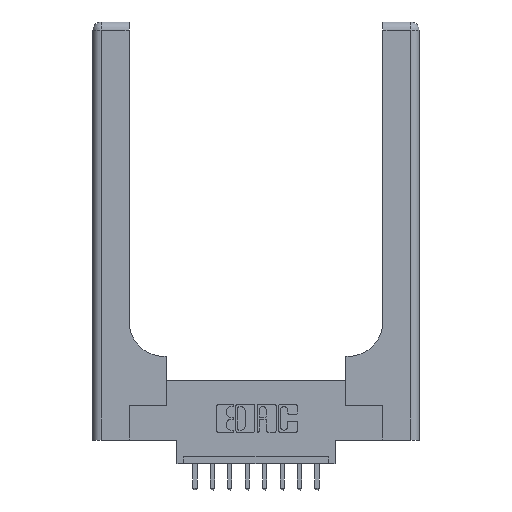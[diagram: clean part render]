
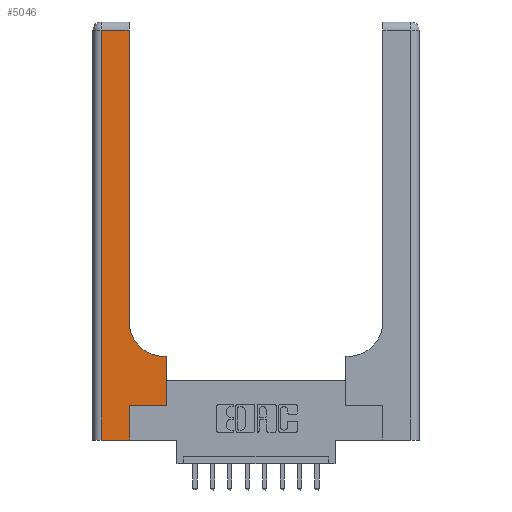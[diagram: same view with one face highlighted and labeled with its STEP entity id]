
A CAD part, top view. The second image highlights one B-rep face of the part: STEP entity #5046.
In plain terms, the highlighted planar face has unit normal (0, 0, 1).
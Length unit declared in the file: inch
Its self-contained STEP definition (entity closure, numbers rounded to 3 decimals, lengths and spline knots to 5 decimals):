
#338 = DIRECTION ( 'NONE',  ( 0., 0., -1. ) ) ;
#442 = ORIENTED_EDGE ( 'NONE', *, *, #2772, .T. ) ;
#544 = ORIENTED_EDGE ( 'NONE', *, *, #5323, .T. ) ;
#589 = VERTEX_POINT ( 'NONE', #1016 ) ;
#874 = VECTOR ( 'NONE', #15366, 39.37008 ) ;
#1016 = CARTESIAN_POINT ( 'NONE',  ( 0.51, 0.6, 0.37 ) ) ;
#1327 = DIRECTION ( 'NONE',  ( 1., 0., 0. ) ) ;
#1485 = VERTEX_POINT ( 'NONE', #12090 ) ;
#1653 = LINE ( 'NONE', #7400, #7604 ) ;
#1821 = VERTEX_POINT ( 'NONE', #3574 ) ;
#2405 = CARTESIAN_POINT ( 'NONE',  ( 0.265, 0.25, 0.37 ) ) ;
#2482 = LINE ( 'NONE', #2405, #5642 ) ;
#2516 = DIRECTION ( 'NONE',  ( 1., 0., 0. ) ) ;
#2554 = CARTESIAN_POINT ( 'NONE',  ( 0.528, 0.25, 0.37 ) ) ;
#2682 = LINE ( 'NONE', #13598, #6756 ) ;
#2772 = EDGE_CURVE ( 'NONE', #6327, #9045, #2682, .T. ) ;
#2813 = DIRECTION ( 'NONE',  ( 0., -1., 0. ) ) ;
#3048 = EDGE_CURVE ( 'NONE', #14672, #6327, #8404, .T. ) ;
#3568 = ORIENTED_EDGE ( 'NONE', *, *, #6844, .T. ) ;
#3574 = CARTESIAN_POINT ( 'NONE',  ( 0.528, 0.6, 0.37 ) ) ;
#3576 = CARTESIAN_POINT ( 'NONE',  ( 0.26, 0.6, 0.37 ) ) ;
#3763 = PLANE ( 'NONE',  #12555 ) ;
#4080 = VECTOR ( 'NONE', #7355, 39.37008 ) ;
#4128 = CARTESIAN_POINT ( 'NONE',  ( 0.06, 3., 0.37 ) ) ;
#4358 = LINE ( 'NONE', #15286, #874 ) ;
#4708 = EDGE_CURVE ( 'NONE', #6042, #1485, #11103, .T. ) ;
#4834 = CARTESIAN_POINT ( 'NONE',  ( 0.51, 0.85, 0.37 ) ) ;
#5046 = ADVANCED_FACE ( 'NONE', ( #13121 ), #3763, .F. ) ;
#5095 = EDGE_CURVE ( 'NONE', #589, #6042, #13806, .T. ) ;
#5323 = EDGE_CURVE ( 'NONE', #1485, #5506, #4358, .T. ) ;
#5395 = CARTESIAN_POINT ( 'NONE',  ( 0.26, 0.85, 0.37 ) ) ;
#5506 = VERTEX_POINT ( 'NONE', #12083 ) ;
#5523 = ORIENTED_EDGE ( 'NONE', *, *, #8245, .T. ) ;
#5611 = ORIENTED_EDGE ( 'NONE', *, *, #9095, .T. ) ;
#5642 = VECTOR ( 'NONE', #8316, 39.37008 ) ;
#5799 = AXIS2_PLACEMENT_3D ( 'NONE', #4834, #338, #2516 ) ;
#6042 = VERTEX_POINT ( 'NONE', #5395 ) ;
#6134 = CARTESIAN_POINT ( 'NONE',  ( 0., 0., 0.37 ) ) ;
#6182 = CARTESIAN_POINT ( 'NONE',  ( 0.26, 3., 0.37 ) ) ;
#6327 = VERTEX_POINT ( 'NONE', #11086 ) ;
#6462 = DIRECTION ( 'NONE',  ( 0., 1., 0. ) ) ;
#6603 = VECTOR ( 'NONE', #2813, 39.37008 ) ;
#6622 = VECTOR ( 'NONE', #9346, 39.37008 ) ;
#6756 = VECTOR ( 'NONE', #8603, 39.37008 ) ;
#6844 = EDGE_CURVE ( 'NONE', #5506, #14672, #14823, .T. ) ;
#7149 = ORIENTED_EDGE ( 'NONE', *, *, #4708, .T. ) ;
#7355 = DIRECTION ( 'NONE',  ( 0., 1., 0. ) ) ;
#7400 = CARTESIAN_POINT ( 'NONE',  ( 0.528, 0.25, 0.37 ) ) ;
#7604 = VECTOR ( 'NONE', #6462, 39.37008 ) ;
#8245 = EDGE_CURVE ( 'NONE', #9045, #13779, #2482, .T. ) ;
#8316 = DIRECTION ( 'NONE',  ( 1., 0., 0. ) ) ;
#8404 = LINE ( 'NONE', #6134, #12280 ) ;
#8603 = DIRECTION ( 'NONE',  ( 0., 1., 0. ) ) ;
#9045 = VERTEX_POINT ( 'NONE', #9976 ) ;
#9095 = EDGE_CURVE ( 'NONE', #13779, #1821, #1653, .T. ) ;
#9346 = DIRECTION ( 'NONE',  ( -1., 0., 0. ) ) ;
#9354 = EDGE_CURVE ( 'NONE', #1821, #589, #14265, .T. ) ;
#9761 = DIRECTION ( 'NONE',  ( -1., 0., 0. ) ) ;
#9976 = CARTESIAN_POINT ( 'NONE',  ( 0.265, 0.25, 0.37 ) ) ;
#10163 = ORIENTED_EDGE ( 'NONE', *, *, #3048, .T. ) ;
#11009 = DIRECTION ( 'NONE',  ( 0., 0., -1. ) ) ;
#11086 = CARTESIAN_POINT ( 'NONE',  ( 0.265, 0., 0.37 ) ) ;
#11103 = LINE ( 'NONE', #6182, #4080 ) ;
#11455 = EDGE_LOOP ( 'NONE', ( #7149, #544, #3568, #10163, #442, #5523, #5611, #14997, #14273 ) ) ;
#12083 = CARTESIAN_POINT ( 'NONE',  ( 0.06, 2.94, 0.37 ) ) ;
#12090 = CARTESIAN_POINT ( 'NONE',  ( 0.26, 2.94, 0.37 ) ) ;
#12280 = VECTOR ( 'NONE', #1327, 39.37008 ) ;
#12555 = AXIS2_PLACEMENT_3D ( 'NONE', #14295, #11009, #9761 ) ;
#13121 = FACE_OUTER_BOUND ( 'NONE', #11455, .T. ) ;
#13598 = CARTESIAN_POINT ( 'NONE',  ( 0.265, 0., 0.37 ) ) ;
#13779 = VERTEX_POINT ( 'NONE', #2554 ) ;
#13806 = CIRCLE ( 'NONE', #5799, 0.25 ) ;
#14265 = LINE ( 'NONE', #3576, #6622 ) ;
#14273 = ORIENTED_EDGE ( 'NONE', *, *, #5095, .T. ) ;
#14295 = CARTESIAN_POINT ( 'NONE',  ( 0., 3., 0.37 ) ) ;
#14459 = CARTESIAN_POINT ( 'NONE',  ( 0.06, 0., 0.37 ) ) ;
#14672 = VERTEX_POINT ( 'NONE', #14459 ) ;
#14823 = LINE ( 'NONE', #4128, #6603 ) ;
#14997 = ORIENTED_EDGE ( 'NONE', *, *, #9354, .T. ) ;
#15286 = CARTESIAN_POINT ( 'NONE',  ( 0., 2.94, 0.37 ) ) ;
#15366 = DIRECTION ( 'NONE',  ( -1., 0., 0. ) ) ;
